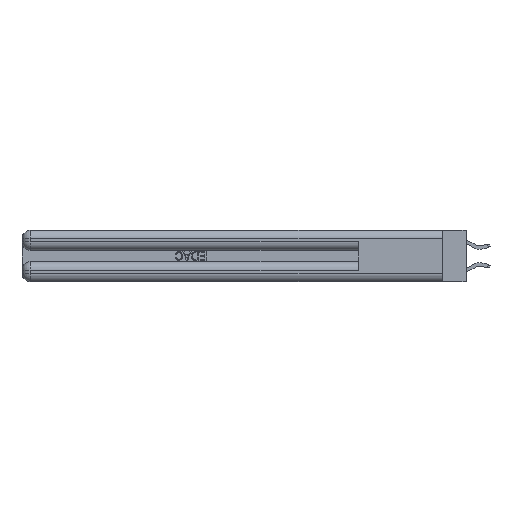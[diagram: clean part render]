
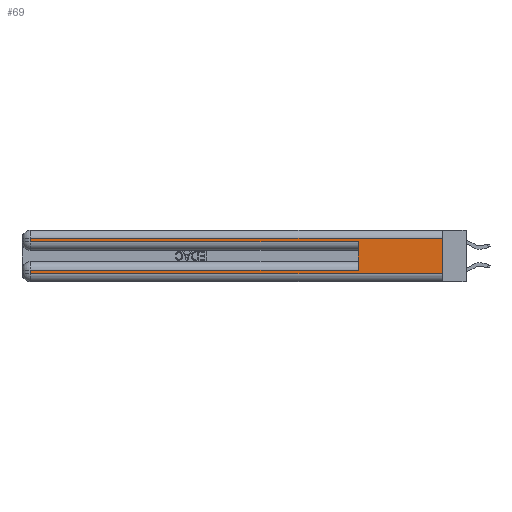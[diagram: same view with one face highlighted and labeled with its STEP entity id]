
A CAD part, left-side view. The second image highlights one B-rep face of the part: STEP entity #69.
In plain terms, the highlighted planar face has unit normal (-1, 0, 0).
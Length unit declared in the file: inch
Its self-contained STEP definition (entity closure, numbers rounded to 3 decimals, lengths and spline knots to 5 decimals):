
#69 = ADVANCED_FACE ( 'NONE', ( #14190 ), #9967, .F. ) ;
#329 = VERTEX_POINT ( 'NONE', #7042 ) ;
#442 = EDGE_CURVE ( 'NONE', #21923, #8271, #9643, .T. ) ;
#655 = DIRECTION ( 'NONE',  ( 0., 1., 0. ) ) ;
#1141 = VECTOR ( 'NONE', #8809, 39.37008 ) ;
#2411 = VERTEX_POINT ( 'NONE', #12195 ) ;
#2739 = LINE ( 'NONE', #18322, #3600 ) ;
#3087 = VERTEX_POINT ( 'NONE', #3619 ) ;
#3600 = VECTOR ( 'NONE', #27165, 39.37008 ) ;
#3619 = CARTESIAN_POINT ( 'NONE',  ( 0., 0.6, 0.085 ) ) ;
#3623 = LINE ( 'NONE', #19062, #26812 ) ;
#3752 = ORIENTED_EDGE ( 'NONE', *, *, #4168, .F. ) ;
#3995 = VECTOR ( 'NONE', #20757, 39.37008 ) ;
#4168 = EDGE_CURVE ( 'NONE', #3087, #2411, #3623, .T. ) ;
#4379 = ORIENTED_EDGE ( 'NONE', *, *, #26756, .T. ) ;
#4774 = LINE ( 'NONE', #18021, #3995 ) ;
#5459 = DIRECTION ( 'NONE',  ( 0., 0., -1. ) ) ;
#5465 = VECTOR ( 'NONE', #27528, 39.37008 ) ;
#6673 = ORIENTED_EDGE ( 'NONE', *, *, #25453, .T. ) ;
#7042 = CARTESIAN_POINT ( 'NONE',  ( 0., 2.94, 0.085 ) ) ;
#7063 = VECTOR ( 'NONE', #23043, 39.37008 ) ;
#7113 = LINE ( 'NONE', #24852, #25893 ) ;
#7167 = ORIENTED_EDGE ( 'NONE', *, *, #26887, .T. ) ;
#8171 = EDGE_CURVE ( 'NONE', #3087, #329, #20443, .T. ) ;
#8172 = ORIENTED_EDGE ( 'NONE', *, *, #8171, .T. ) ;
#8271 = VERTEX_POINT ( 'NONE', #17073 ) ;
#8479 = CARTESIAN_POINT ( 'NONE',  ( 0., 0., 0.06 ) ) ;
#8722 = VERTEX_POINT ( 'NONE', #27941 ) ;
#8758 = VERTEX_POINT ( 'NONE', #12244 ) ;
#8809 = DIRECTION ( 'NONE',  ( 0., -1., 0. ) ) ;
#9434 = EDGE_CURVE ( 'NONE', #8722, #2411, #10599, .T. ) ;
#9643 = LINE ( 'NONE', #13880, #5465 ) ;
#9967 = PLANE ( 'NONE',  #11096 ) ;
#10599 = LINE ( 'NONE', #17703, #1141 ) ;
#11096 = AXIS2_PLACEMENT_3D ( 'NONE', #16527, #25377, #5459 ) ;
#11147 = VERTEX_POINT ( 'NONE', #20602 ) ;
#12195 = CARTESIAN_POINT ( 'NONE',  ( 0., 0.6, 0.285 ) ) ;
#12244 = CARTESIAN_POINT ( 'NONE',  ( 0., 2.94, 0.06 ) ) ;
#13880 = CARTESIAN_POINT ( 'NONE',  ( 0., 0., 0.37 ) ) ;
#14176 = CARTESIAN_POINT ( 'NONE',  ( 0., 0., 0.085 ) ) ;
#14190 = FACE_OUTER_BOUND ( 'NONE', #22149, .T. ) ;
#15744 = VECTOR ( 'NONE', #15777, 39.37008 ) ;
#15777 = DIRECTION ( 'NONE',  ( 0., -1., 0. ) ) ;
#16527 = CARTESIAN_POINT ( 'NONE',  ( 0., 0., 0.37 ) ) ;
#17073 = CARTESIAN_POINT ( 'NONE',  ( 0., 0., 0.06 ) ) ;
#17512 = LINE ( 'NONE', #8479, #15744 ) ;
#17703 = CARTESIAN_POINT ( 'NONE',  ( 0., 0., 0.285 ) ) ;
#18021 = CARTESIAN_POINT ( 'NONE',  ( 0., 2.94, 0.37 ) ) ;
#18322 = CARTESIAN_POINT ( 'NONE',  ( 0., 2.94, 0.37 ) ) ;
#19062 = CARTESIAN_POINT ( 'NONE',  ( 0., 0.6, 0.145 ) ) ;
#19315 = ORIENTED_EDGE ( 'NONE', *, *, #9434, .T. ) ;
#20443 = LINE ( 'NONE', #14176, #7063 ) ;
#20602 = CARTESIAN_POINT ( 'NONE',  ( 0., 2.94, 0.31 ) ) ;
#20680 = ORIENTED_EDGE ( 'NONE', *, *, #27262, .T. ) ;
#20757 = DIRECTION ( 'NONE',  ( 0., 0., -1. ) ) ;
#21923 = VERTEX_POINT ( 'NONE', #26616 ) ;
#22149 = EDGE_LOOP ( 'NONE', ( #26570, #7167, #6673, #19315, #3752, #8172, #4379, #20680 ) ) ;
#23043 = DIRECTION ( 'NONE',  ( 0., 1., 0. ) ) ;
#24852 = CARTESIAN_POINT ( 'NONE',  ( 0., 0., 0.31 ) ) ;
#25377 = DIRECTION ( 'NONE',  ( 1., 0., 0. ) ) ;
#25449 = DIRECTION ( 'NONE',  ( 0., 0., 1. ) ) ;
#25453 = EDGE_CURVE ( 'NONE', #11147, #8722, #4774, .T. ) ;
#25893 = VECTOR ( 'NONE', #655, 39.37008 ) ;
#26570 = ORIENTED_EDGE ( 'NONE', *, *, #442, .F. ) ;
#26616 = CARTESIAN_POINT ( 'NONE',  ( 0., 0., 0.31 ) ) ;
#26756 = EDGE_CURVE ( 'NONE', #329, #8758, #2739, .T. ) ;
#26812 = VECTOR ( 'NONE', #25449, 39.37008 ) ;
#26887 = EDGE_CURVE ( 'NONE', #21923, #11147, #7113, .T. ) ;
#27165 = DIRECTION ( 'NONE',  ( 0., 0., -1. ) ) ;
#27262 = EDGE_CURVE ( 'NONE', #8758, #8271, #17512, .T. ) ;
#27528 = DIRECTION ( 'NONE',  ( 0., 0., -1. ) ) ;
#27941 = CARTESIAN_POINT ( 'NONE',  ( 0., 2.94, 0.285 ) ) ;
